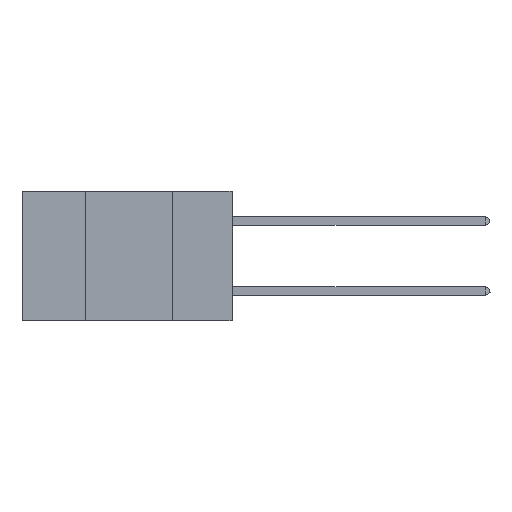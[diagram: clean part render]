
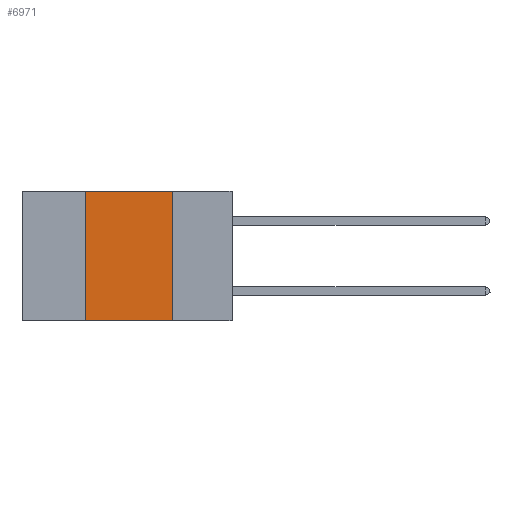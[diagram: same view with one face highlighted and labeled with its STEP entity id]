
A CAD part, left-side view. The second image highlights one B-rep face of the part: STEP entity #6971.
In plain terms, the highlighted planar face has unit normal (-1, 0, 0).
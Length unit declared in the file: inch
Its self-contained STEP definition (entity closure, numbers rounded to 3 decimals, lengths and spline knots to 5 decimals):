
#484 = EDGE_CURVE ( 'NONE', #19250, #36411, #1116, .T. ) ;
#609 = CARTESIAN_POINT ( 'NONE',  ( 0., 0.17, 0. ) ) ;
#1116 = LINE ( 'NONE', #25443, #14108 ) ;
#2731 = DIRECTION ( 'NONE',  ( 0., 0., -1. ) ) ;
#4505 = FACE_OUTER_BOUND ( 'NONE', #13600, .T. ) ;
#5461 = EDGE_CURVE ( 'NONE', #19250, #22664, #27110, .T. ) ;
#6971 = ADVANCED_FACE ( 'NONE', ( #4505 ), #12511, .F. ) ;
#7983 = CARTESIAN_POINT ( 'NONE',  ( 0., 0.6, -0.37 ) ) ;
#8963 = CARTESIAN_POINT ( 'NONE',  ( 0., 0.17, 0. ) ) ;
#9445 = CARTESIAN_POINT ( 'NONE',  ( 0., 0.17, -0.37 ) ) ;
#10256 = DIRECTION ( 'NONE',  ( 0., 0., -1. ) ) ;
#12136 = VECTOR ( 'NONE', #26851, 39.37008 ) ;
#12244 = ORIENTED_EDGE ( 'NONE', *, *, #5461, .T. ) ;
#12511 = PLANE ( 'NONE',  #25214 ) ;
#13600 = EDGE_LOOP ( 'NONE', ( #34572, #24441, #15692, #12244 ) ) ;
#13777 = LINE ( 'NONE', #609, #28704 ) ;
#14095 = EDGE_CURVE ( 'NONE', #31123, #22664, #13777, .T. ) ;
#14108 = VECTOR ( 'NONE', #32515, 39.37008 ) ;
#15692 = ORIENTED_EDGE ( 'NONE', *, *, #484, .F. ) ;
#16492 = CARTESIAN_POINT ( 'NONE',  ( 0., 0.42, 0. ) ) ;
#16810 = CARTESIAN_POINT ( 'NONE',  ( 0., 0.42, -0.37 ) ) ;
#17127 = CARTESIAN_POINT ( 'NONE',  ( 0., 0.6, 0. ) ) ;
#19250 = VERTEX_POINT ( 'NONE', #16810 ) ;
#21556 = EDGE_CURVE ( 'NONE', #36411, #31123, #37257, .T. ) ;
#21867 = DIRECTION ( 'NONE',  ( 1., 0., 0. ) ) ;
#22664 = VERTEX_POINT ( 'NONE', #9445 ) ;
#24441 = ORIENTED_EDGE ( 'NONE', *, *, #21556, .F. ) ;
#25214 = AXIS2_PLACEMENT_3D ( 'NONE', #28253, #21867, #2731 ) ;
#25443 = CARTESIAN_POINT ( 'NONE',  ( 0., 0.42, 0. ) ) ;
#26851 = DIRECTION ( 'NONE',  ( 0., -1., 0. ) ) ;
#27110 = LINE ( 'NONE', #7983, #12136 ) ;
#28253 = CARTESIAN_POINT ( 'NONE',  ( 0., 0.6, 0. ) ) ;
#28704 = VECTOR ( 'NONE', #10256, 39.37008 ) ;
#31123 = VERTEX_POINT ( 'NONE', #8963 ) ;
#32515 = DIRECTION ( 'NONE',  ( 0., 0., 1. ) ) ;
#32740 = VECTOR ( 'NONE', #35684, 39.37008 ) ;
#34572 = ORIENTED_EDGE ( 'NONE', *, *, #14095, .F. ) ;
#35684 = DIRECTION ( 'NONE',  ( 0., -1., 0. ) ) ;
#36411 = VERTEX_POINT ( 'NONE', #16492 ) ;
#37257 = LINE ( 'NONE', #17127, #32740 ) ;
